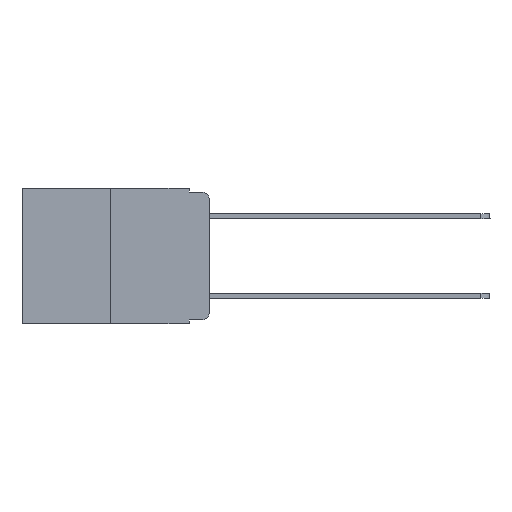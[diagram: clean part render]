
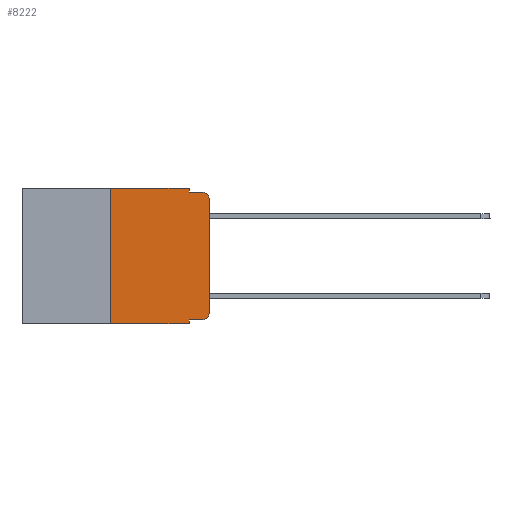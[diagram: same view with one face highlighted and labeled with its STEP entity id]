
A CAD part, left-side view. The second image highlights one B-rep face of the part: STEP entity #8222.
In plain terms, the highlighted planar face has unit normal (-1, 0, 0).
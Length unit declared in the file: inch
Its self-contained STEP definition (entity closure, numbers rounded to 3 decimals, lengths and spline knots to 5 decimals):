
#575 = VERTEX_POINT ( 'NONE', #10116 ) ;
#638 = CARTESIAN_POINT ( 'NONE',  ( 0., 0.051, 0. ) ) ;
#682 = LINE ( 'NONE', #8000, #13949 ) ;
#743 = EDGE_CURVE ( 'NONE', #3018, #6897, #18159, .T. ) ;
#1193 = VECTOR ( 'NONE', #13950, 39.37008 ) ;
#1713 = DIRECTION ( 'NONE',  ( 0., 0., -1. ) ) ;
#1729 = FACE_OUTER_BOUND ( 'NONE', #8019, .T. ) ;
#1935 = DIRECTION ( 'NONE',  ( 0., -1., 0. ) ) ;
#2185 = VERTEX_POINT ( 'NONE', #9392 ) ;
#2272 = DIRECTION ( 'NONE',  ( 0., 0., 1. ) ) ;
#2450 = AXIS2_PLACEMENT_3D ( 'NONE', #7949, #7809, #19796 ) ;
#2460 = EDGE_CURVE ( 'NONE', #20817, #2874, #4193, .T. ) ;
#2874 = VERTEX_POINT ( 'NONE', #7917 ) ;
#3018 = VERTEX_POINT ( 'NONE', #11844 ) ;
#3533 = CARTESIAN_POINT ( 'NONE',  ( 0., 0.02, -0.03 ) ) ;
#3640 = ORIENTED_EDGE ( 'NONE', *, *, #743, .T. ) ;
#4193 = LINE ( 'NONE', #17362, #1193 ) ;
#4265 = PLANE ( 'NONE',  #16765 ) ;
#4758 = EDGE_CURVE ( 'NONE', #5833, #8973, #21683, .T. ) ;
#5019 = CARTESIAN_POINT ( 'NONE',  ( 0., 0., -0.03 ) ) ;
#5833 = VERTEX_POINT ( 'NONE', #10037 ) ;
#6024 = ORIENTED_EDGE ( 'NONE', *, *, #10259, .F. ) ;
#6553 = EDGE_CURVE ( 'NONE', #19436, #5833, #16466, .T. ) ;
#6562 = VERTEX_POINT ( 'NONE', #14032 ) ;
#6897 = VERTEX_POINT ( 'NONE', #5019 ) ;
#6973 = CARTESIAN_POINT ( 'NONE',  ( 0., 0.25, 0. ) ) ;
#7442 = DIRECTION ( 'NONE',  ( 1., 0., 0. ) ) ;
#7627 = VECTOR ( 'NONE', #12746, 39.37008 ) ;
#7809 = DIRECTION ( 'NONE',  ( -1., 0., 0. ) ) ;
#7917 = CARTESIAN_POINT ( 'NONE',  ( 0., 0.051, -0.343 ) ) ;
#7949 = CARTESIAN_POINT ( 'NONE',  ( 0., 0.02, -0.313 ) ) ;
#8000 = CARTESIAN_POINT ( 'NONE',  ( 0., 0.051, -0.333 ) ) ;
#8019 = EDGE_LOOP ( 'NONE', ( #3640, #20237, #19609, #14343, #13753, #17681, #15137, #6024, #18228, #17665 ) ) ;
#8156 = VECTOR ( 'NONE', #18356, 39.37008 ) ;
#8222 = ADVANCED_FACE ( 'NONE', ( #1729 ), #4265, .F. ) ;
#8240 = EDGE_CURVE ( 'NONE', #20817, #19436, #21752, .T. ) ;
#8448 = AXIS2_PLACEMENT_3D ( 'NONE', #3533, #8638, #1713 ) ;
#8638 = DIRECTION ( 'NONE',  ( -1., 0., 0. ) ) ;
#8973 = VERTEX_POINT ( 'NONE', #18014 ) ;
#9373 = DIRECTION ( 'NONE',  ( 0., 0., 1. ) ) ;
#9392 = CARTESIAN_POINT ( 'NONE',  ( 0., 0.051, -0.333 ) ) ;
#9594 = CARTESIAN_POINT ( 'NONE',  ( 0., 0.25, -0.343 ) ) ;
#10037 = CARTESIAN_POINT ( 'NONE',  ( 0., 0.051, 0. ) ) ;
#10116 = CARTESIAN_POINT ( 'NONE',  ( 0., 0.02, -0.333 ) ) ;
#10259 = EDGE_CURVE ( 'NONE', #2185, #2874, #21928, .T. ) ;
#10624 = CARTESIAN_POINT ( 'NONE',  ( 0., 0.051, -0.01 ) ) ;
#10736 = CIRCLE ( 'NONE', #8448, 0.02 ) ;
#10979 = DIRECTION ( 'NONE',  ( 0., 0., -1. ) ) ;
#11203 = EDGE_CURVE ( 'NONE', #575, #3018, #14576, .T. ) ;
#11844 = CARTESIAN_POINT ( 'NONE',  ( 0., 0., -0.313 ) ) ;
#11886 = VECTOR ( 'NONE', #1935, 39.37008 ) ;
#12746 = DIRECTION ( 'NONE',  ( 0., 0., -1. ) ) ;
#13122 = DIRECTION ( 'NONE',  ( 0., -1., 0. ) ) ;
#13406 = EDGE_CURVE ( 'NONE', #6897, #6562, #10736, .T. ) ;
#13701 = EDGE_CURVE ( 'NONE', #2185, #575, #682, .T. ) ;
#13753 = ORIENTED_EDGE ( 'NONE', *, *, #6553, .F. ) ;
#13949 = VECTOR ( 'NONE', #13122, 39.37008 ) ;
#13950 = DIRECTION ( 'NONE',  ( 0., -1., 0. ) ) ;
#14032 = CARTESIAN_POINT ( 'NONE',  ( 0., 0.02, -0.01 ) ) ;
#14343 = ORIENTED_EDGE ( 'NONE', *, *, #4758, .F. ) ;
#14454 = VECTOR ( 'NONE', #19455, 39.37008 ) ;
#14576 = CIRCLE ( 'NONE', #2450, 0.02 ) ;
#14974 = VECTOR ( 'NONE', #2272, 39.37008 ) ;
#15137 = ORIENTED_EDGE ( 'NONE', *, *, #2460, .T. ) ;
#16345 = LINE ( 'NONE', #10624, #14454 ) ;
#16346 = CARTESIAN_POINT ( 'NONE',  ( 0., 0.473, 0. ) ) ;
#16466 = LINE ( 'NONE', #20849, #11886 ) ;
#16676 = CARTESIAN_POINT ( 'NONE',  ( 0., 0., 0. ) ) ;
#16765 = AXIS2_PLACEMENT_3D ( 'NONE', #16346, #7442, #10979 ) ;
#17362 = CARTESIAN_POINT ( 'NONE',  ( 0., 0.473, -0.343 ) ) ;
#17637 = EDGE_CURVE ( 'NONE', #8973, #6562, #16345, .T. ) ;
#17665 = ORIENTED_EDGE ( 'NONE', *, *, #11203, .T. ) ;
#17681 = ORIENTED_EDGE ( 'NONE', *, *, #8240, .F. ) ;
#17704 = CARTESIAN_POINT ( 'NONE',  ( 0., 0.25, 0. ) ) ;
#18014 = CARTESIAN_POINT ( 'NONE',  ( 0., 0.051, -0.01 ) ) ;
#18159 = LINE ( 'NONE', #16676, #21669 ) ;
#18228 = ORIENTED_EDGE ( 'NONE', *, *, #13701, .T. ) ;
#18356 = DIRECTION ( 'NONE',  ( 0., 0., -1. ) ) ;
#19436 = VERTEX_POINT ( 'NONE', #6973 ) ;
#19455 = DIRECTION ( 'NONE',  ( 0., -1., 0. ) ) ;
#19609 = ORIENTED_EDGE ( 'NONE', *, *, #17637, .F. ) ;
#19796 = DIRECTION ( 'NONE',  ( 0., 0., -1. ) ) ;
#20237 = ORIENTED_EDGE ( 'NONE', *, *, #13406, .T. ) ;
#20244 = CARTESIAN_POINT ( 'NONE',  ( 0., 0.051, 0. ) ) ;
#20817 = VERTEX_POINT ( 'NONE', #9594 ) ;
#20849 = CARTESIAN_POINT ( 'NONE',  ( 0., 0.473, 0. ) ) ;
#21669 = VECTOR ( 'NONE', #9373, 39.37008 ) ;
#21683 = LINE ( 'NONE', #638, #7627 ) ;
#21752 = LINE ( 'NONE', #17704, #14974 ) ;
#21928 = LINE ( 'NONE', #20244, #8156 ) ;
